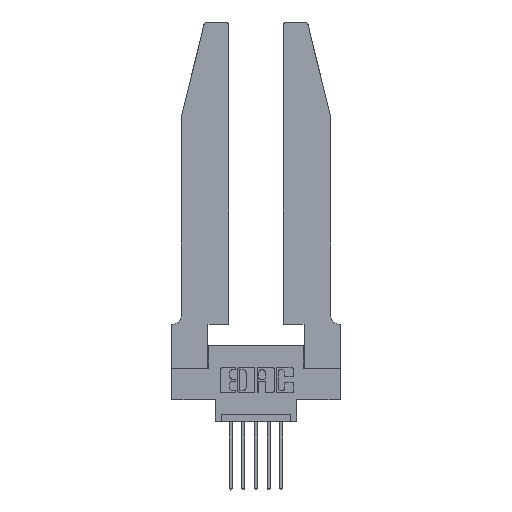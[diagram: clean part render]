
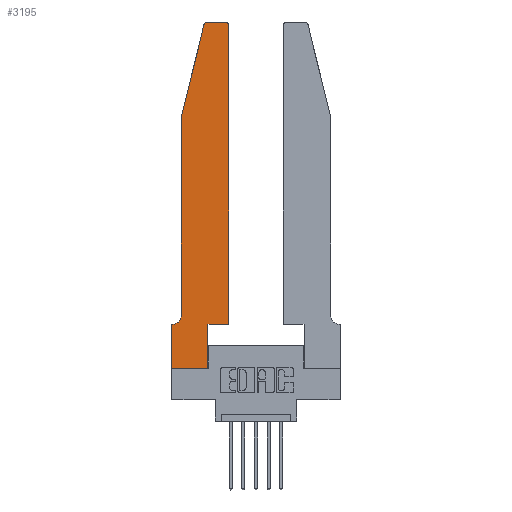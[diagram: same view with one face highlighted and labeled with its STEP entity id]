
A CAD part, top view. The second image highlights one B-rep face of the part: STEP entity #3195.
In plain terms, the highlighted planar face has unit normal (0, 0, 1).
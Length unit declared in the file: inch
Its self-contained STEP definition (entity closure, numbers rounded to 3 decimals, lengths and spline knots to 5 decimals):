
#6 = LINE ( 'NONE', #8948, #12704 ) ;
#526 = LINE ( 'NONE', #1156, #13212 ) ;
#566 = CARTESIAN_POINT ( 'NONE',  ( 0.0055, 0.42, 0.37 ) ) ;
#622 = CARTESIAN_POINT ( 'NONE',  ( 0., 0., 0.37 ) ) ;
#779 = LINE ( 'NONE', #6422, #13117 ) ;
#1156 = CARTESIAN_POINT ( 'NONE',  ( 0.4505, 0.35, 0.37 ) ) ;
#1165 = EDGE_CURVE ( 'NONE', #8449, #1735, #13118, .T. ) ;
#1305 = EDGE_CURVE ( 'NONE', #3333, #13367, #6856, .T. ) ;
#1627 = EDGE_CURVE ( 'NONE', #7358, #12269, #526, .T. ) ;
#1735 = VERTEX_POINT ( 'NONE', #5111 ) ;
#1795 = EDGE_CURVE ( 'NONE', #4851, #7406, #1861, .T. ) ;
#1861 = LINE ( 'NONE', #7294, #4345 ) ;
#1913 = EDGE_CURVE ( 'NONE', #13367, #4851, #6441, .T. ) ;
#2092 = EDGE_CURVE ( 'NONE', #8238, #13098, #6, .T. ) ;
#2225 = ORIENTED_EDGE ( 'NONE', *, *, #2658, .T. ) ;
#2385 = CARTESIAN_POINT ( 'NONE',  ( 0.4505, 0.35, 0.37 ) ) ;
#2658 = EDGE_CURVE ( 'NONE', #5421, #8449, #8560, .T. ) ;
#2975 = LINE ( 'NONE', #9144, #5279 ) ;
#3085 = PLANE ( 'NONE',  #12056 ) ;
#3195 = ADVANCED_FACE ( 'NONE', ( #10692 ), #3085, .T. ) ;
#3333 = VERTEX_POINT ( 'NONE', #12769 ) ;
#3677 = VECTOR ( 'NONE', #6908, 39.37008 ) ;
#3790 = DIRECTION ( 'NONE',  ( 0., 0., -1. ) ) ;
#3838 = ORIENTED_EDGE ( 'NONE', *, *, #1305, .T. ) ;
#3867 = CARTESIAN_POINT ( 'NONE',  ( 0.4505, 0.35, 0.37 ) ) ;
#4047 = VECTOR ( 'NONE', #9735, 39.37008 ) ;
#4281 = CARTESIAN_POINT ( 'NONE',  ( 0.4205, 2.72, 0.37 ) ) ;
#4328 = VECTOR ( 'NONE', #9553, 39.37008 ) ;
#4331 = CARTESIAN_POINT ( 'NONE',  ( 0.284, 2.75, 0.37 ) ) ;
#4334 = ORIENTED_EDGE ( 'NONE', *, *, #1165, .T. ) ;
#4345 = VECTOR ( 'NONE', #6167, 39.37008 ) ;
#4381 = CARTESIAN_POINT ( 'NONE',  ( 0.4505, 2.72, 0.37 ) ) ;
#4514 = DIRECTION ( 'NONE',  ( 1., 0., 0. ) ) ;
#4642 = ORIENTED_EDGE ( 'NONE', *, *, #1795, .T. ) ;
#4851 = VERTEX_POINT ( 'NONE', #7750 ) ;
#4951 = ORIENTED_EDGE ( 'NONE', *, *, #9990, .T. ) ;
#5001 = ORIENTED_EDGE ( 'NONE', *, *, #12399, .T. ) ;
#5111 = CARTESIAN_POINT ( 'NONE',  ( 0.25487, 2.72718, 0.37 ) ) ;
#5129 = ORIENTED_EDGE ( 'NONE', *, *, #11371, .T. ) ;
#5279 = VECTOR ( 'NONE', #11302, 39.37008 ) ;
#5409 = CARTESIAN_POINT ( 'NONE',  ( 0.0055, 0.35, 0.37 ) ) ;
#5418 = AXIS2_PLACEMENT_3D ( 'NONE', #10743, #9636, #4514 ) ;
#5421 = VERTEX_POINT ( 'NONE', #5792 ) ;
#5792 = CARTESIAN_POINT ( 'NONE',  ( 0.4205, 2.75, 0.37 ) ) ;
#6146 = CARTESIAN_POINT ( 'NONE',  ( 0.2865, 0.35, 0.37 ) ) ;
#6152 = DIRECTION ( 'NONE',  ( 1., 0., 0. ) ) ;
#6167 = DIRECTION ( 'NONE',  ( 0., -1., 0. ) ) ;
#6179 = ORIENTED_EDGE ( 'NONE', *, *, #1627, .T. ) ;
#6422 = CARTESIAN_POINT ( 'NONE',  ( 0.0755, 2., 0.37 ) ) ;
#6441 = LINE ( 'NONE', #11721, #4328 ) ;
#6802 = LINE ( 'NONE', #2385, #4047 ) ;
#6856 = CIRCLE ( 'NONE', #9910, 0.07 ) ;
#6908 = DIRECTION ( 'NONE',  ( -0.239, -0.971, 0. ) ) ;
#7120 = ORIENTED_EDGE ( 'NONE', *, *, #2092, .T. ) ;
#7294 = CARTESIAN_POINT ( 'NONE',  ( 0., 0., 0.37 ) ) ;
#7358 = VERTEX_POINT ( 'NONE', #3867 ) ;
#7406 = VERTEX_POINT ( 'NONE', #622 ) ;
#7750 = CARTESIAN_POINT ( 'NONE',  ( 0., 0.35, 0.37 ) ) ;
#7888 = CIRCLE ( 'NONE', #12273, 0.03 ) ;
#7983 = DIRECTION ( 'NONE',  ( 0., 1., 0. ) ) ;
#8080 = CARTESIAN_POINT ( 'NONE',  ( 0.2865, 0., 0.37 ) ) ;
#8238 = VERTEX_POINT ( 'NONE', #8080 ) ;
#8268 = ORIENTED_EDGE ( 'NONE', *, *, #1913, .T. ) ;
#8390 = CARTESIAN_POINT ( 'NONE',  ( 0., 0.35, 0.37 ) ) ;
#8441 = EDGE_CURVE ( 'NONE', #8767, #3333, #779, .T. ) ;
#8449 = VERTEX_POINT ( 'NONE', #4331 ) ;
#8560 = LINE ( 'NONE', #11787, #11527 ) ;
#8699 = ORIENTED_EDGE ( 'NONE', *, *, #12564, .T. ) ;
#8767 = VERTEX_POINT ( 'NONE', #11606 ) ;
#8933 = DIRECTION ( 'NONE',  ( -1., 0., 0. ) ) ;
#8948 = CARTESIAN_POINT ( 'NONE',  ( 0.2865, 0.35, 0.37 ) ) ;
#8979 = CARTESIAN_POINT ( 'NONE',  ( 0.0755, 2., 0.37 ) ) ;
#9144 = CARTESIAN_POINT ( 'NONE',  ( 0., 0., 0.37 ) ) ;
#9355 = DIRECTION ( 'NONE',  ( 0., 0., 1. ) ) ;
#9491 = DIRECTION ( 'NONE',  ( 0., -1., 0. ) ) ;
#9553 = DIRECTION ( 'NONE',  ( -1., 0., 0. ) ) ;
#9636 = DIRECTION ( 'NONE',  ( 0., 0., 1. ) ) ;
#9735 = DIRECTION ( 'NONE',  ( 1., 0., 0. ) ) ;
#9769 = ORIENTED_EDGE ( 'NONE', *, *, #8441, .T. ) ;
#9904 = EDGE_LOOP ( 'NONE', ( #2225, #4334, #5129, #9769, #3838, #8268, #4642, #5001, #7120, #4951, #6179, #8699 ) ) ;
#9910 = AXIS2_PLACEMENT_3D ( 'NONE', #566, #3790, #8933 ) ;
#9990 = EDGE_CURVE ( 'NONE', #13098, #7358, #6802, .T. ) ;
#10692 = FACE_OUTER_BOUND ( 'NONE', #9904, .T. ) ;
#10725 = DIRECTION ( 'NONE',  ( 0., 1., 0. ) ) ;
#10743 = CARTESIAN_POINT ( 'NONE',  ( 0.284, 2.72, 0.37 ) ) ;
#10817 = DIRECTION ( 'NONE',  ( -1., 0., 0. ) ) ;
#11302 = DIRECTION ( 'NONE',  ( 1., 0., 0. ) ) ;
#11371 = EDGE_CURVE ( 'NONE', #1735, #8767, #11861, .T. ) ;
#11526 = DIRECTION ( 'NONE',  ( 1., 0., 0. ) ) ;
#11527 = VECTOR ( 'NONE', #10817, 39.37008 ) ;
#11606 = CARTESIAN_POINT ( 'NONE',  ( 0.0755, 2., 0.37 ) ) ;
#11614 = DIRECTION ( 'NONE',  ( 0., 0., 1. ) ) ;
#11721 = CARTESIAN_POINT ( 'NONE',  ( 0.0755, 0.35, 0.37 ) ) ;
#11787 = CARTESIAN_POINT ( 'NONE',  ( 0.2605, 2.75, 0.37 ) ) ;
#11861 = LINE ( 'NONE', #8979, #3677 ) ;
#12056 = AXIS2_PLACEMENT_3D ( 'NONE', #8390, #9355, #11526 ) ;
#12269 = VERTEX_POINT ( 'NONE', #4381 ) ;
#12273 = AXIS2_PLACEMENT_3D ( 'NONE', #4281, #11614, #6152 ) ;
#12399 = EDGE_CURVE ( 'NONE', #7406, #8238, #2975, .T. ) ;
#12564 = EDGE_CURVE ( 'NONE', #12269, #5421, #7888, .T. ) ;
#12704 = VECTOR ( 'NONE', #7983, 39.37008 ) ;
#12769 = CARTESIAN_POINT ( 'NONE',  ( 0.0755, 0.42, 0.37 ) ) ;
#13098 = VERTEX_POINT ( 'NONE', #6146 ) ;
#13117 = VECTOR ( 'NONE', #9491, 39.37008 ) ;
#13118 = CIRCLE ( 'NONE', #5418, 0.03 ) ;
#13212 = VECTOR ( 'NONE', #10725, 39.37008 ) ;
#13367 = VERTEX_POINT ( 'NONE', #5409 ) ;
